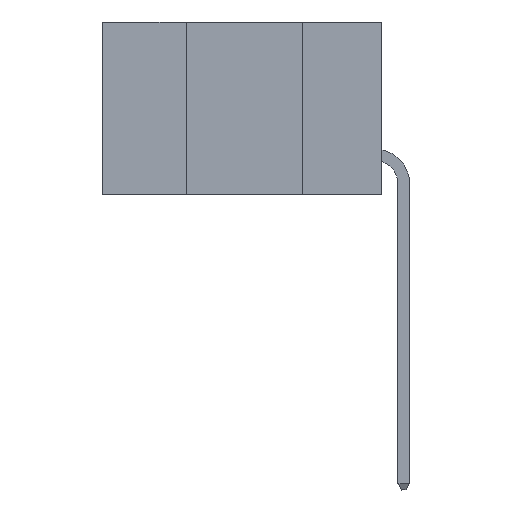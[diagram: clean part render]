
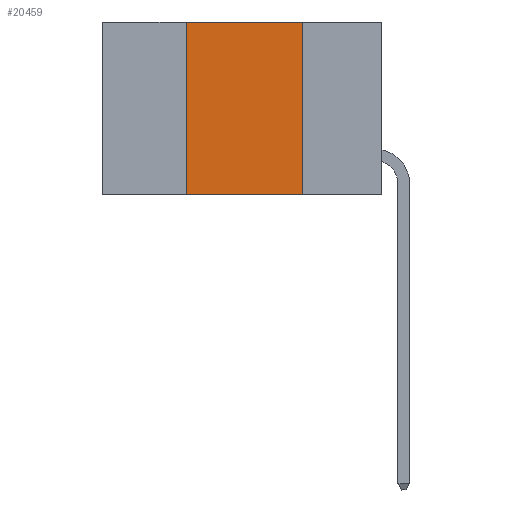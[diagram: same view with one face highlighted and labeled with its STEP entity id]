
A CAD part, left-side view. The second image highlights one B-rep face of the part: STEP entity #20459.
In plain terms, the highlighted planar face has unit normal (-1, 0, 0).
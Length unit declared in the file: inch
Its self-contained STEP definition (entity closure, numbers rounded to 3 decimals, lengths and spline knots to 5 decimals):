
#440 = AXIS2_PLACEMENT_3D ( 'NONE', #13872, #20911, #27305 ) ;
#1473 = ORIENTED_EDGE ( 'NONE', *, *, #8355, .F. ) ;
#1679 = CARTESIAN_POINT ( 'NONE',  ( 0., 0.6, -0.37 ) ) ;
#1771 = EDGE_CURVE ( 'NONE', #13174, #13334, #16490, .T. ) ;
#3405 = CARTESIAN_POINT ( 'NONE',  ( 0., 0.42, 0. ) ) ;
#4391 = CARTESIAN_POINT ( 'NONE',  ( 0., 0.17, 0. ) ) ;
#8355 = EDGE_CURVE ( 'NONE', #27035, #27979, #21418, .T. ) ;
#8460 = VECTOR ( 'NONE', #9997, 39.37008 ) ;
#8608 = EDGE_CURVE ( 'NONE', #27035, #13334, #21062, .T. ) ;
#8630 = VECTOR ( 'NONE', #21554, 39.37008 ) ;
#9293 = PLANE ( 'NONE',  #440 ) ;
#9997 = DIRECTION ( 'NONE',  ( 0., -1., 0. ) ) ;
#11826 = CARTESIAN_POINT ( 'NONE',  ( 0., 0.17, 0. ) ) ;
#12355 = DIRECTION ( 'NONE',  ( 0., 0., 1. ) ) ;
#13126 = FACE_OUTER_BOUND ( 'NONE', #24292, .T. ) ;
#13174 = VERTEX_POINT ( 'NONE', #11826 ) ;
#13334 = VERTEX_POINT ( 'NONE', #20543 ) ;
#13872 = CARTESIAN_POINT ( 'NONE',  ( 0., 0.6, 0. ) ) ;
#16490 = LINE ( 'NONE', #4391, #8630 ) ;
#17006 = VECTOR ( 'NONE', #28008, 39.37008 ) ;
#17284 = EDGE_CURVE ( 'NONE', #27979, #13174, #24411, .T. ) ;
#19524 = CARTESIAN_POINT ( 'NONE',  ( 0., 0.42, -0.37 ) ) ;
#20148 = CARTESIAN_POINT ( 'NONE',  ( 0., 0.42, 0. ) ) ;
#20459 = ADVANCED_FACE ( 'NONE', ( #13126 ), #9293, .F. ) ;
#20543 = CARTESIAN_POINT ( 'NONE',  ( 0., 0.17, -0.37 ) ) ;
#20911 = DIRECTION ( 'NONE',  ( 1., 0., 0. ) ) ;
#21062 = LINE ( 'NONE', #1679, #8460 ) ;
#21369 = ORIENTED_EDGE ( 'NONE', *, *, #8608, .T. ) ;
#21418 = LINE ( 'NONE', #3405, #24726 ) ;
#21554 = DIRECTION ( 'NONE',  ( 0., 0., -1. ) ) ;
#22045 = ORIENTED_EDGE ( 'NONE', *, *, #1771, .F. ) ;
#22140 = CARTESIAN_POINT ( 'NONE',  ( 0., 0.6, 0. ) ) ;
#24292 = EDGE_LOOP ( 'NONE', ( #22045, #24688, #1473, #21369 ) ) ;
#24411 = LINE ( 'NONE', #22140, #17006 ) ;
#24688 = ORIENTED_EDGE ( 'NONE', *, *, #17284, .F. ) ;
#24726 = VECTOR ( 'NONE', #12355, 39.37008 ) ;
#27035 = VERTEX_POINT ( 'NONE', #19524 ) ;
#27305 = DIRECTION ( 'NONE',  ( 0., 0., -1. ) ) ;
#27979 = VERTEX_POINT ( 'NONE', #20148 ) ;
#28008 = DIRECTION ( 'NONE',  ( 0., -1., 0. ) ) ;
